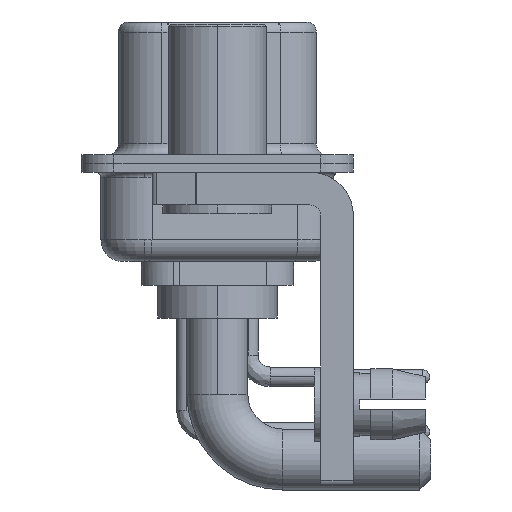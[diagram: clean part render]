
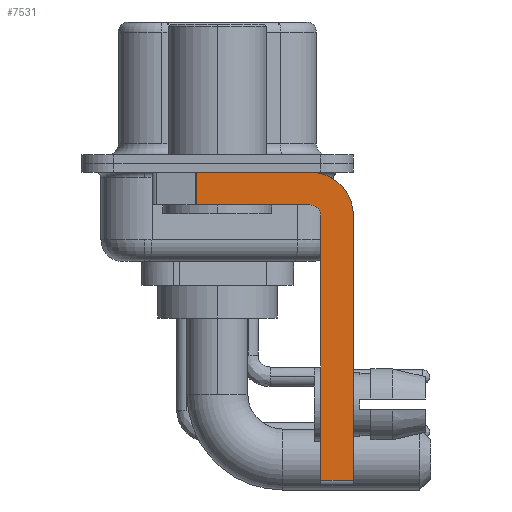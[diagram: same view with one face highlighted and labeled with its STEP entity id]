
A CAD part, left-side view. The second image highlights one B-rep face of the part: STEP entity #7531.
In plain terms, the highlighted planar face has unit normal (-1, 0, 0).
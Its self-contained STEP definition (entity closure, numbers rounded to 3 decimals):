
#19 = DIRECTION ( 'NONE',  ( 0., 0., -1. ) ) ;
#258 = CIRCLE ( 'NONE', #12042, 0.5 ) ;
#1095 = AXIS2_PLACEMENT_3D ( 'NONE', #22600, #24532, #19 ) ;
#1134 = EDGE_CURVE ( 'NONE', #20689, #2493, #6614, .T. ) ;
#1915 = VECTOR ( 'NONE', #6647, 1000. ) ;
#2493 = VERTEX_POINT ( 'NONE', #12974 ) ;
#2594 = ORIENTED_EDGE ( 'NONE', *, *, #6070, .T. ) ;
#3416 = ORIENTED_EDGE ( 'NONE', *, *, #28930, .F. ) ;
#4015 = CARTESIAN_POINT ( 'NONE',  ( -2.9, -6.25, -2.4 ) ) ;
#4243 = DIRECTION ( 'NONE',  ( 0., 0., 1. ) ) ;
#4602 = DIRECTION ( 'NONE',  ( 0., 0., -1. ) ) ;
#4736 = PLANE ( 'NONE',  #1095 ) ;
#5808 = CARTESIAN_POINT ( 'NONE',  ( -2.9, -4.25, -1.9 ) ) ;
#6070 = EDGE_CURVE ( 'NONE', #11826, #16650, #11344, .T. ) ;
#6310 = VECTOR ( 'NONE', #26613, 1000. ) ;
#6614 = LINE ( 'NONE', #21811, #18750 ) ;
#6647 = DIRECTION ( 'NONE',  ( 0., -1., 0. ) ) ;
#7211 = CARTESIAN_POINT ( 'NONE',  ( -2.9, -4.25, -1.9 ) ) ;
#7531 = ADVANCED_FACE ( 'NONE', ( #24965 ), #4736, .F. ) ;
#7737 = CARTESIAN_POINT ( 'NONE',  ( -2.9, 0.978, -0.4 ) ) ;
#8488 = DIRECTION ( 'NONE',  ( 0., -1., 0. ) ) ;
#8614 = AXIS2_PLACEMENT_3D ( 'NONE', #25081, #17975, #22565 ) ;
#9152 = CARTESIAN_POINT ( 'NONE',  ( -2.9, 3., -0.4 ) ) ;
#9268 = EDGE_CURVE ( 'NONE', #24727, #24167, #21346, .T. ) ;
#9576 = VERTEX_POINT ( 'NONE', #25369 ) ;
#9907 = CARTESIAN_POINT ( 'NONE',  ( -2.9, 0.978, -1.9 ) ) ;
#10366 = DIRECTION ( 'NONE',  ( 0., 0., 1. ) ) ;
#10668 = CARTESIAN_POINT ( 'NONE',  ( -2.9, -4.25, -2.4 ) ) ;
#10790 = ORIENTED_EDGE ( 'NONE', *, *, #16230, .F. ) ;
#10796 = EDGE_CURVE ( 'NONE', #24167, #9576, #13323, .T. ) ;
#10809 = DIRECTION ( 'NONE',  ( -1., 0., 0. ) ) ;
#10931 = LINE ( 'NONE', #9152, #1915 ) ;
#11297 = ORIENTED_EDGE ( 'NONE', *, *, #11486, .T. ) ;
#11303 = EDGE_LOOP ( 'NONE', ( #14580, #2594, #3416, #10790, #16451, #11297, #21278, #21430 ) ) ;
#11344 = LINE ( 'NONE', #23003, #24612 ) ;
#11486 = EDGE_CURVE ( 'NONE', #20689, #9576, #19681, .T. ) ;
#11826 = VERTEX_POINT ( 'NONE', #7737 ) ;
#12042 = AXIS2_PLACEMENT_3D ( 'NONE', #10668, #10809, #10366 ) ;
#12742 = LINE ( 'NONE', #5808, #6310 ) ;
#12974 = CARTESIAN_POINT ( 'NONE',  ( -2.9, -4.75, -2.4 ) ) ;
#13323 = LINE ( 'NONE', #17870, #22039 ) ;
#13926 = CARTESIAN_POINT ( 'NONE',  ( -2.9, -4.25, -0.4 ) ) ;
#14580 = ORIENTED_EDGE ( 'NONE', *, *, #26019, .F. ) ;
#16230 = EDGE_CURVE ( 'NONE', #2493, #22929, #258, .T. ) ;
#16451 = ORIENTED_EDGE ( 'NONE', *, *, #1134, .F. ) ;
#16650 = VERTEX_POINT ( 'NONE', #9907 ) ;
#17870 = CARTESIAN_POINT ( 'NONE',  ( -2.9, -6.25, -2.4 ) ) ;
#17975 = DIRECTION ( 'NONE',  ( 1., 0., 0. ) ) ;
#18750 = VECTOR ( 'NONE', #4243, 1000. ) ;
#19681 = LINE ( 'NONE', #28719, #19843 ) ;
#19843 = VECTOR ( 'NONE', #8488, 1000. ) ;
#20176 = DIRECTION ( 'NONE',  ( 0., 0., -1. ) ) ;
#20689 = VERTEX_POINT ( 'NONE', #22582 ) ;
#21278 = ORIENTED_EDGE ( 'NONE', *, *, #10796, .F. ) ;
#21346 = CIRCLE ( 'NONE', #8614, 2. ) ;
#21430 = ORIENTED_EDGE ( 'NONE', *, *, #9268, .F. ) ;
#21811 = CARTESIAN_POINT ( 'NONE',  ( -2.9, -4.75, -14.8 ) ) ;
#22039 = VECTOR ( 'NONE', #4602, 1000. ) ;
#22565 = DIRECTION ( 'NONE',  ( 0., 0., -1. ) ) ;
#22582 = CARTESIAN_POINT ( 'NONE',  ( -2.9, -4.75, -14.55 ) ) ;
#22600 = CARTESIAN_POINT ( 'NONE',  ( -2.9, -4.25, -2.4 ) ) ;
#22929 = VERTEX_POINT ( 'NONE', #7211 ) ;
#23003 = CARTESIAN_POINT ( 'NONE',  ( -2.9, 0.978, -1.9 ) ) ;
#24167 = VERTEX_POINT ( 'NONE', #4015 ) ;
#24532 = DIRECTION ( 'NONE',  ( 1., 0., 0. ) ) ;
#24612 = VECTOR ( 'NONE', #20176, 1000. ) ;
#24727 = VERTEX_POINT ( 'NONE', #13926 ) ;
#24965 = FACE_OUTER_BOUND ( 'NONE', #11303, .T. ) ;
#25081 = CARTESIAN_POINT ( 'NONE',  ( -2.9, -4.25, -2.4 ) ) ;
#25369 = CARTESIAN_POINT ( 'NONE',  ( -2.9, -6.25, -14.55 ) ) ;
#26019 = EDGE_CURVE ( 'NONE', #11826, #24727, #10931, .T. ) ;
#26613 = DIRECTION ( 'NONE',  ( 0., 1., 0. ) ) ;
#28719 = CARTESIAN_POINT ( 'NONE',  ( -2.9, -4.25, -14.55 ) ) ;
#28930 = EDGE_CURVE ( 'NONE', #22929, #16650, #12742, .T. ) ;
